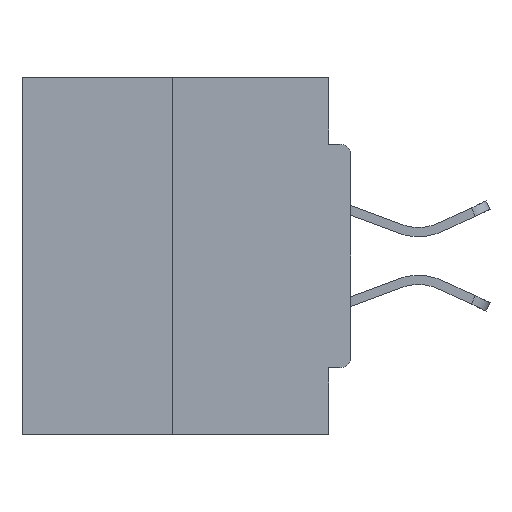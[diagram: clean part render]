
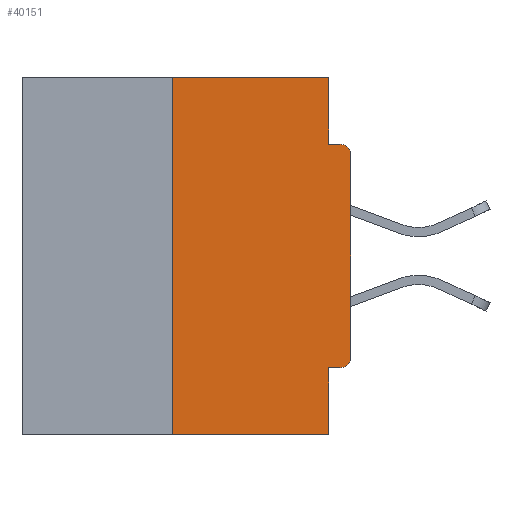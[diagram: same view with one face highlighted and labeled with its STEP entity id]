
A CAD part, left-side view. The second image highlights one B-rep face of the part: STEP entity #40151.
In plain terms, the highlighted planar face has unit normal (-1, 0, 0).
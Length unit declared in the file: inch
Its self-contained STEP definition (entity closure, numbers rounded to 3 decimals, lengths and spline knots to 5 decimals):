
#14 = VERTEX_POINT ( 'NONE', #3182 ) ;
#309 = VERTEX_POINT ( 'NONE', #8054 ) ;
#432 = VERTEX_POINT ( 'NONE', #2519 ) ;
#1074 = EDGE_CURVE ( 'NONE', #432, #12213, #40771, .T. ) ;
#2519 = CARTESIAN_POINT ( 'NONE',  ( 0., 0.015, -0.4065 ) ) ;
#2985 = DIRECTION ( 'NONE',  ( 0., 0., 1. ) ) ;
#3182 = CARTESIAN_POINT ( 'NONE',  ( 0., 0., -0.1085 ) ) ;
#3339 = VECTOR ( 'NONE', #16962, 39.37008 ) ;
#3435 = EDGE_LOOP ( 'NONE', ( #9521, #8185, #15592, #14324, #7342, #5742, #17432, #27336, #11763, #12899 ) ) ;
#3793 = VERTEX_POINT ( 'NONE', #26551 ) ;
#5190 = DIRECTION ( 'NONE',  ( -1., 0., 0. ) ) ;
#5267 = EDGE_CURVE ( 'NONE', #16192, #9574, #28509, .T. ) ;
#5742 = ORIENTED_EDGE ( 'NONE', *, *, #1074, .T. ) ;
#6021 = LINE ( 'NONE', #13246, #34798 ) ;
#6139 = PLANE ( 'NONE',  #41624 ) ;
#6328 = DIRECTION ( 'NONE',  ( 0., 0., -1. ) ) ;
#6557 = EDGE_CURVE ( 'NONE', #9574, #24164, #42944, .T. ) ;
#7116 = AXIS2_PLACEMENT_3D ( 'NONE', #38361, #5190, #41970 ) ;
#7342 = ORIENTED_EDGE ( 'NONE', *, *, #37544, .F. ) ;
#7430 = CARTESIAN_POINT ( 'NONE',  ( 0., 0.46, 0. ) ) ;
#7860 = VERTEX_POINT ( 'NONE', #21654 ) ;
#8054 = CARTESIAN_POINT ( 'NONE',  ( 0., 0.031, -0.4065 ) ) ;
#8160 = LINE ( 'NONE', #21512, #38527 ) ;
#8185 = ORIENTED_EDGE ( 'NONE', *, *, #5267, .F. ) ;
#8467 = CARTESIAN_POINT ( 'NONE',  ( 0., 0.25, -0.5 ) ) ;
#9089 = LINE ( 'NONE', #35023, #24352 ) ;
#9225 = VERTEX_POINT ( 'NONE', #37604 ) ;
#9521 = ORIENTED_EDGE ( 'NONE', *, *, #6557, .F. ) ;
#9574 = VERTEX_POINT ( 'NONE', #26352 ) ;
#9576 = DIRECTION ( 'NONE',  ( 0., -1., 0. ) ) ;
#11341 = LINE ( 'NONE', #12659, #26585 ) ;
#11763 = ORIENTED_EDGE ( 'NONE', *, *, #36520, .F. ) ;
#12213 = VERTEX_POINT ( 'NONE', #23591 ) ;
#12386 = DIRECTION ( 'NONE',  ( 0., 0., -1. ) ) ;
#12400 = EDGE_CURVE ( 'NONE', #16192, #3793, #6021, .T. ) ;
#12659 = CARTESIAN_POINT ( 'NONE',  ( 0., 0., 0. ) ) ;
#12822 = DIRECTION ( 'NONE',  ( 1., 0., 0. ) ) ;
#12899 = ORIENTED_EDGE ( 'NONE', *, *, #41161, .F. ) ;
#13246 = CARTESIAN_POINT ( 'NONE',  ( 0., 0.46, -0.5 ) ) ;
#13395 = DIRECTION ( 'NONE',  ( 0., 0., 1. ) ) ;
#14324 = ORIENTED_EDGE ( 'NONE', *, *, #18157, .F. ) ;
#14509 = LINE ( 'NONE', #37071, #19206 ) ;
#15059 = EDGE_CURVE ( 'NONE', #14, #7860, #28830, .T. ) ;
#15592 = ORIENTED_EDGE ( 'NONE', *, *, #12400, .T. ) ;
#16192 = VERTEX_POINT ( 'NONE', #8467 ) ;
#16690 = DIRECTION ( 'NONE',  ( -1., 0., 0. ) ) ;
#16962 = DIRECTION ( 'NONE',  ( 0., 1., 0. ) ) ;
#17432 = ORIENTED_EDGE ( 'NONE', *, *, #33279, .T. ) ;
#18157 = EDGE_CURVE ( 'NONE', #309, #3793, #8160, .T. ) ;
#18273 = DIRECTION ( 'NONE',  ( 0., 0., -1. ) ) ;
#19206 = VECTOR ( 'NONE', #40393, 39.37008 ) ;
#20216 = CARTESIAN_POINT ( 'NONE',  ( 0., 0.25, 0. ) ) ;
#21512 = CARTESIAN_POINT ( 'NONE',  ( 0., 0.031, -0.5 ) ) ;
#21654 = CARTESIAN_POINT ( 'NONE',  ( 0., 0.015, -0.0935 ) ) ;
#23443 = AXIS2_PLACEMENT_3D ( 'NONE', #42841, #16690, #6328 ) ;
#23591 = CARTESIAN_POINT ( 'NONE',  ( 0., 0., -0.3915 ) ) ;
#23791 = VECTOR ( 'NONE', #2985, 39.37008 ) ;
#24164 = VERTEX_POINT ( 'NONE', #36586 ) ;
#24352 = VECTOR ( 'NONE', #31405, 39.37008 ) ;
#25755 = CARTESIAN_POINT ( 'NONE',  ( 0., 0.46, 0. ) ) ;
#26352 = CARTESIAN_POINT ( 'NONE',  ( 0., 0.25, 0. ) ) ;
#26551 = CARTESIAN_POINT ( 'NONE',  ( 0., 0.031, -0.5 ) ) ;
#26585 = VECTOR ( 'NONE', #13395, 39.37008 ) ;
#26883 = LINE ( 'NONE', #40040, #3339 ) ;
#27336 = ORIENTED_EDGE ( 'NONE', *, *, #15059, .T. ) ;
#27654 = DIRECTION ( 'NONE',  ( 0., -1., 0. ) ) ;
#28509 = LINE ( 'NONE', #20216, #23791 ) ;
#28830 = CIRCLE ( 'NONE', #7116, 0.015 ) ;
#31405 = DIRECTION ( 'NONE',  ( 0., -1., 0. ) ) ;
#31519 = VECTOR ( 'NONE', #27654, 39.37008 ) ;
#33279 = EDGE_CURVE ( 'NONE', #12213, #14, #11341, .T. ) ;
#34798 = VECTOR ( 'NONE', #9576, 39.37008 ) ;
#35023 = CARTESIAN_POINT ( 'NONE',  ( 0., 0., -0.0935 ) ) ;
#35983 = FACE_OUTER_BOUND ( 'NONE', #3435, .T. ) ;
#36520 = EDGE_CURVE ( 'NONE', #9225, #7860, #9089, .T. ) ;
#36586 = CARTESIAN_POINT ( 'NONE',  ( 0., 0.031, 0. ) ) ;
#37071 = CARTESIAN_POINT ( 'NONE',  ( 0., 0.031, 0. ) ) ;
#37544 = EDGE_CURVE ( 'NONE', #432, #309, #26883, .T. ) ;
#37604 = CARTESIAN_POINT ( 'NONE',  ( 0., 0.031, -0.0935 ) ) ;
#38361 = CARTESIAN_POINT ( 'NONE',  ( 0., 0.015, -0.1085 ) ) ;
#38527 = VECTOR ( 'NONE', #18273, 39.37008 ) ;
#40040 = CARTESIAN_POINT ( 'NONE',  ( 0., 0., -0.4065 ) ) ;
#40151 = ADVANCED_FACE ( 'NONE', ( #35983 ), #6139, .F. ) ;
#40393 = DIRECTION ( 'NONE',  ( 0., 0., -1. ) ) ;
#40771 = CIRCLE ( 'NONE', #23443, 0.015 ) ;
#41161 = EDGE_CURVE ( 'NONE', #24164, #9225, #14509, .T. ) ;
#41624 = AXIS2_PLACEMENT_3D ( 'NONE', #25755, #12822, #12386 ) ;
#41970 = DIRECTION ( 'NONE',  ( 0., 0., -1. ) ) ;
#42841 = CARTESIAN_POINT ( 'NONE',  ( 0., 0.015, -0.3915 ) ) ;
#42944 = LINE ( 'NONE', #7430, #31519 ) ;
